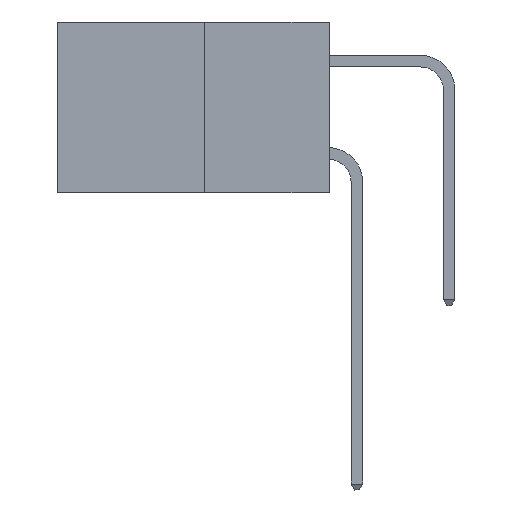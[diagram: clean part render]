
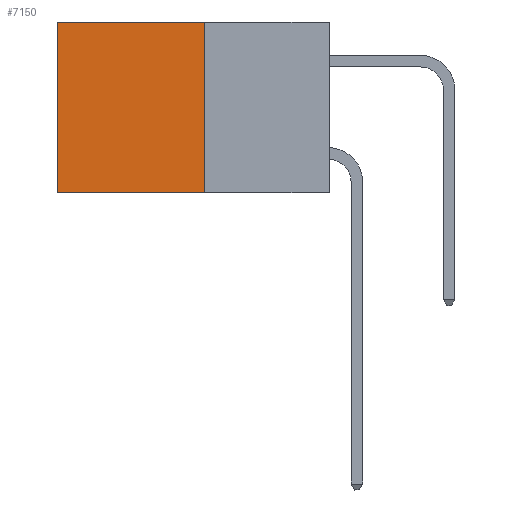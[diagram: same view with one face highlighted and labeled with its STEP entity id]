
A CAD part, left-side view. The second image highlights one B-rep face of the part: STEP entity #7150.
In plain terms, the highlighted planar face has unit normal (-1, 0, 0).
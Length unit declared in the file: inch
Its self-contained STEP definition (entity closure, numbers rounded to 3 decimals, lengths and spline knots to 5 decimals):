
#815 = DIRECTION ( 'NONE',  ( 0., 1., 0. ) ) ;
#1604 = EDGE_LOOP ( 'NONE', ( #6000, #10211, #14401, #19034 ) ) ;
#1909 = PLANE ( 'NONE',  #15489 ) ;
#1960 = DIRECTION ( 'NONE',  ( 0., 0., -1. ) ) ;
#2054 = CARTESIAN_POINT ( 'NONE',  ( 0.277, 0.27, -0.37 ) ) ;
#2851 = CARTESIAN_POINT ( 'NONE',  ( 0.277, 0.59, -0.37 ) ) ;
#3429 = EDGE_CURVE ( 'NONE', #16788, #9999, #19915, .T. ) ;
#5086 = CARTESIAN_POINT ( 'NONE',  ( 0.277, 0.27, -0.37 ) ) ;
#6000 = ORIENTED_EDGE ( 'NONE', *, *, #3429, .T. ) ;
#6551 = VERTEX_POINT ( 'NONE', #7868 ) ;
#7150 = ADVANCED_FACE ( 'NONE', ( #9929 ), #1909, .F. ) ;
#7767 = DIRECTION ( 'NONE',  ( 0., 0., -1. ) ) ;
#7868 = CARTESIAN_POINT ( 'NONE',  ( 0.277, 0.27, 0. ) ) ;
#8595 = VECTOR ( 'NONE', #11759, 39.37008 ) ;
#9116 = DIRECTION ( 'NONE',  ( 1., 0., 0. ) ) ;
#9788 = VECTOR ( 'NONE', #7767, 39.37008 ) ;
#9929 = FACE_OUTER_BOUND ( 'NONE', #1604, .T. ) ;
#9999 = VERTEX_POINT ( 'NONE', #2851 ) ;
#10211 = ORIENTED_EDGE ( 'NONE', *, *, #19728, .F. ) ;
#10341 = EDGE_CURVE ( 'NONE', #6551, #16486, #17640, .T. ) ;
#10440 = VECTOR ( 'NONE', #815, 39.37008 ) ;
#11344 = CARTESIAN_POINT ( 'NONE',  ( 0.277, 0.27, -0.37 ) ) ;
#11759 = DIRECTION ( 'NONE',  ( 0., 0., -1. ) ) ;
#12224 = VECTOR ( 'NONE', #15317, 39.37008 ) ;
#14401 = ORIENTED_EDGE ( 'NONE', *, *, #10341, .F. ) ;
#14476 = LINE ( 'NONE', #17910, #10440 ) ;
#15317 = DIRECTION ( 'NONE',  ( 0., 1., 0. ) ) ;
#15489 = AXIS2_PLACEMENT_3D ( 'NONE', #2054, #9116, #1960 ) ;
#16232 = LINE ( 'NONE', #5086, #12224 ) ;
#16486 = VERTEX_POINT ( 'NONE', #11344 ) ;
#16788 = VERTEX_POINT ( 'NONE', #19749 ) ;
#17640 = LINE ( 'NONE', #19437, #8595 ) ;
#17910 = CARTESIAN_POINT ( 'NONE',  ( 0.277, 0.27, 0. ) ) ;
#18650 = EDGE_CURVE ( 'NONE', #6551, #16788, #14476, .T. ) ;
#19034 = ORIENTED_EDGE ( 'NONE', *, *, #18650, .T. ) ;
#19437 = CARTESIAN_POINT ( 'NONE',  ( 0.277, 0.27, -0.37 ) ) ;
#19728 = EDGE_CURVE ( 'NONE', #16486, #9999, #16232, .T. ) ;
#19749 = CARTESIAN_POINT ( 'NONE',  ( 0.277, 0.59, 0. ) ) ;
#19771 = CARTESIAN_POINT ( 'NONE',  ( 0.277, 0.59, -0.37 ) ) ;
#19915 = LINE ( 'NONE', #19771, #9788 ) ;
